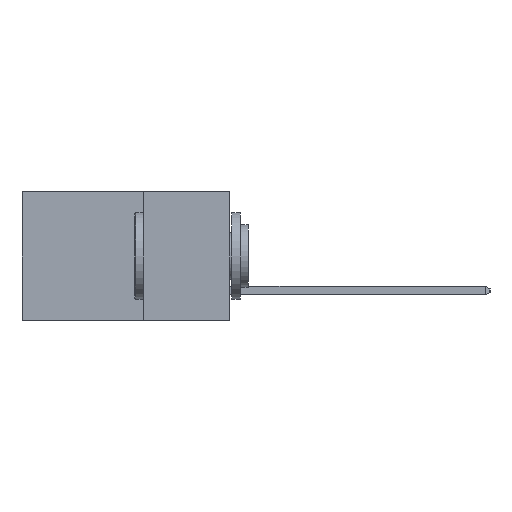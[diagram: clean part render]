
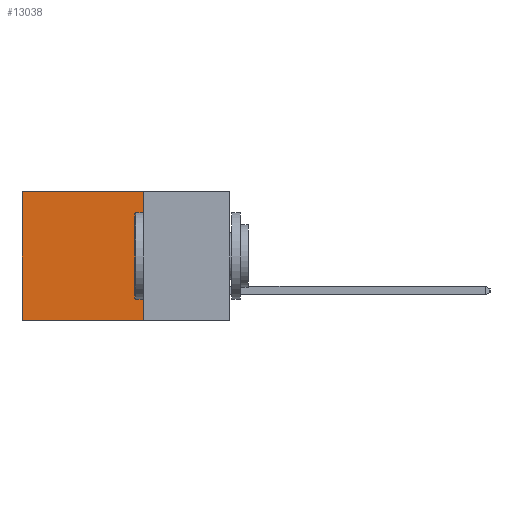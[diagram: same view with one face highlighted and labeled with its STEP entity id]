
A CAD part, left-side view. The second image highlights one B-rep face of the part: STEP entity #13038.
In plain terms, the highlighted planar face has unit normal (-1, 0, 0).
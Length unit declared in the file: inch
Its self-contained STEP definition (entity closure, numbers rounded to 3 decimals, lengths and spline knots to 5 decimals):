
#74 = CARTESIAN_POINT ( 'NONE',  ( 0.2615, 0.6, -0.37 ) ) ;
#1526 = EDGE_LOOP ( 'NONE', ( #25197, #11638, #23500, #18774 ) ) ;
#2265 = LINE ( 'NONE', #74, #22817 ) ;
#2637 = VERTEX_POINT ( 'NONE', #10292 ) ;
#2962 = VECTOR ( 'NONE', #14168, 39.37008 ) ;
#4923 = EDGE_CURVE ( 'NONE', #2637, #10991, #24014, .T. ) ;
#6715 = DIRECTION ( 'NONE',  ( 0., 1., 0. ) ) ;
#6764 = CARTESIAN_POINT ( 'NONE',  ( 0.2615, 0.25, -0.37 ) ) ;
#6877 = DIRECTION ( 'NONE',  ( 0., 0., -1. ) ) ;
#8126 = CARTESIAN_POINT ( 'NONE',  ( 0.2615, 0.6, -0.37 ) ) ;
#8360 = VECTOR ( 'NONE', #17003, 39.37008 ) ;
#8933 = CARTESIAN_POINT ( 'NONE',  ( 0.2615, 0.25, 0. ) ) ;
#10218 = EDGE_CURVE ( 'NONE', #10991, #19041, #18749, .T. ) ;
#10292 = CARTESIAN_POINT ( 'NONE',  ( 0.2615, 0.25, 0. ) ) ;
#10991 = VERTEX_POINT ( 'NONE', #24501 ) ;
#11638 = ORIENTED_EDGE ( 'NONE', *, *, #10218, .F. ) ;
#13038 = ADVANCED_FACE ( 'NONE', ( #14290 ), #14915, .F. ) ;
#14140 = VECTOR ( 'NONE', #6715, 39.37008 ) ;
#14168 = DIRECTION ( 'NONE',  ( 0., 0., -1. ) ) ;
#14290 = FACE_OUTER_BOUND ( 'NONE', #1526, .T. ) ;
#14346 = CARTESIAN_POINT ( 'NONE',  ( 0.2615, 0.25, -0.37 ) ) ;
#14915 = PLANE ( 'NONE',  #15032 ) ;
#15032 = AXIS2_PLACEMENT_3D ( 'NONE', #16872, #18852, #6877 ) ;
#15165 = VERTEX_POINT ( 'NONE', #21076 ) ;
#16254 = DIRECTION ( 'NONE',  ( 0., 0., -1. ) ) ;
#16872 = CARTESIAN_POINT ( 'NONE',  ( 0.2615, 0.25, -0.37 ) ) ;
#17003 = DIRECTION ( 'NONE',  ( 0., 1., 0. ) ) ;
#18749 = LINE ( 'NONE', #6764, #14140 ) ;
#18774 = ORIENTED_EDGE ( 'NONE', *, *, #22876, .T. ) ;
#18852 = DIRECTION ( 'NONE',  ( 1., 0., 0. ) ) ;
#19041 = VERTEX_POINT ( 'NONE', #8126 ) ;
#21076 = CARTESIAN_POINT ( 'NONE',  ( 0.2615, 0.6, 0. ) ) ;
#22817 = VECTOR ( 'NONE', #16254, 39.37008 ) ;
#22876 = EDGE_CURVE ( 'NONE', #2637, #15165, #24065, .T. ) ;
#23500 = ORIENTED_EDGE ( 'NONE', *, *, #4923, .F. ) ;
#24014 = LINE ( 'NONE', #14346, #2962 ) ;
#24065 = LINE ( 'NONE', #8933, #8360 ) ;
#24501 = CARTESIAN_POINT ( 'NONE',  ( 0.2615, 0.25, -0.37 ) ) ;
#24993 = EDGE_CURVE ( 'NONE', #15165, #19041, #2265, .T. ) ;
#25197 = ORIENTED_EDGE ( 'NONE', *, *, #24993, .T. ) ;
